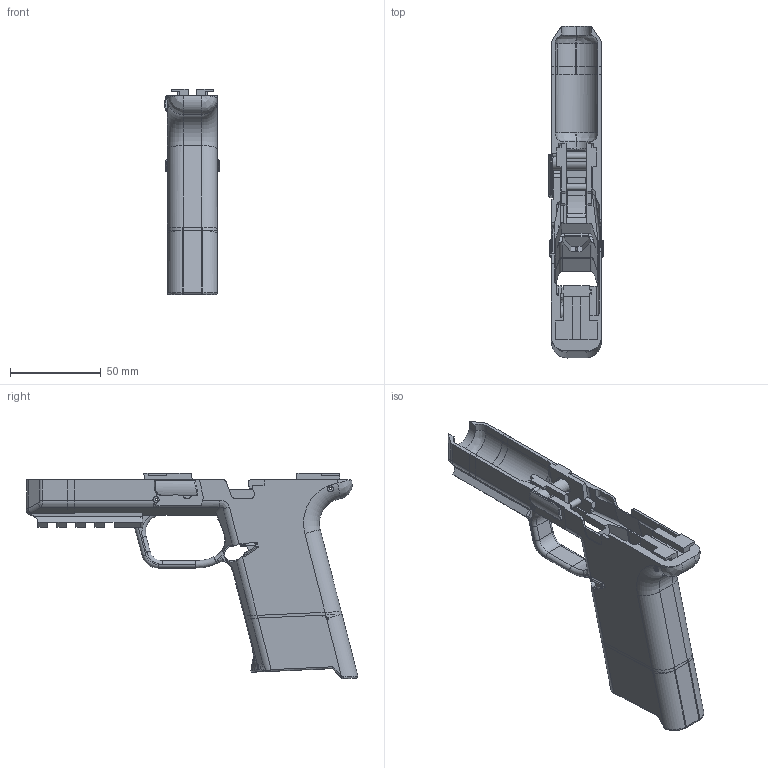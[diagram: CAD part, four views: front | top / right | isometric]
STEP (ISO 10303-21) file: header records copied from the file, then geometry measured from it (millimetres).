
FILE_DESCRIPTION(/* description */ (''),/* implementation_level */ '2;1');
FILE_NAME(/* name */ 'M&P 9 Assembly + Picatinny - Full Size Slide M2.0.step',/* time_stamp */ '2022-02-26T19:45:01-05:00',/* author */ (''),/* organization */ (''),/* preprocessor_version */ 'ST-DEVELOPER v18.1',/* originating_system */ 'Autodesk Translation Framework v10.13.0.1454',/* authorisation */ '');
FILE_SCHEMA (('AUTOMOTIVE_DESIGN { 1 0 10303 214 3 1 1 }'));
Length unit declared in the file: millimetre
Products named in the file (13): M&P 9 M2.0 Standard Length Slide - Picatinny; M&P 9 Reference v117; Rear Fire Control Group Pin; Front Locking Block Group Pin; Trigger Pin; Locking Block; Disassembly Lug; Rear Fire Control Group; Frame; Trigger Guard and Magwell; Fitment Section; M1.0 Full-size Nose; Full-Size Magwell Body
Assembly tree (12 placements, depth 5):
  M&P 9 M2.0 Standard Length Slide - Picatinny
    M&P 9 Reference v117
      Rear Fire Control Group Pin
      Front Locking Block Group Pin
      Trigger Pin
      Locking Block
      Disassembly Lug
      Rear Fire Control Group
      Frame
        Trigger Guard and Magwell
        Fitment Section
          M1.0 Full-size Nose
        Full-Size Magwell Body
Bounding box: 30.21 x 182.43 x 113.13 mm (x, y, z)
Volume: 108913 mm3; surface area: 60500 mm2
Topology: 12 solids, 12 shells, 696 faces, 1888 edges, 1199 vertices
Faces by surface type: plane 361, cylinder 196, bspline 112, torus 21, sphere 4, cone 2
Full cylindrical faces by diameter (mm): 1.35 x2, 1.5 x3, 3.15 x2, 3.18 x3, 3.2 x2, 3.361 x2, 3.5 x1, 3.55 x4, 4.7 x1, 5.1 x1, 6.3 x1, 7.7 x1, 8.8 x1, 9 x2
Entity records: 25868 total; most frequent: CARTESIAN_POINT 8291, ORIENTED_EDGE 3754, DIRECTION 3400, EDGE_CURVE 1877, VERTEX_POINT 1199, LINE 1146, VECTOR 1146, AXIS2_PLACEMENT_3D 1127
